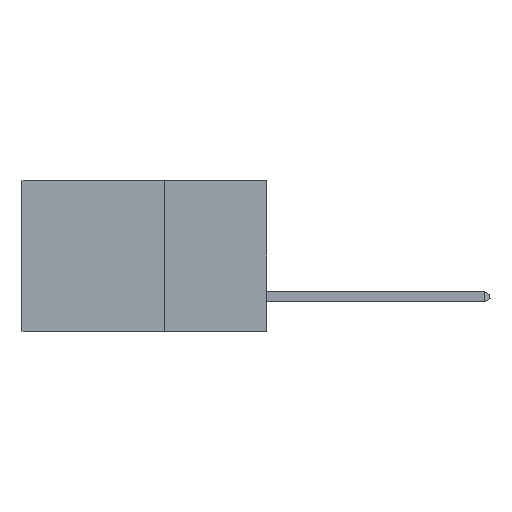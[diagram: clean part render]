
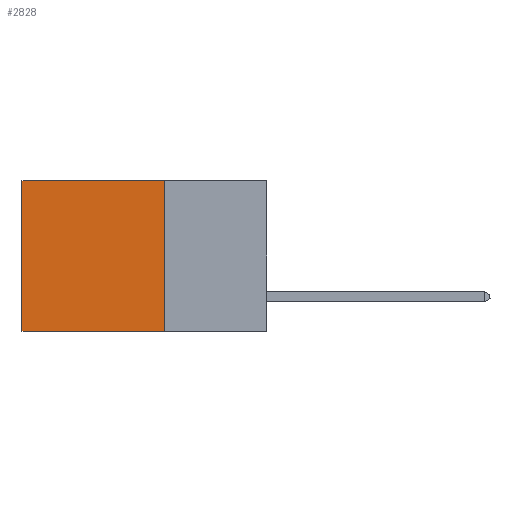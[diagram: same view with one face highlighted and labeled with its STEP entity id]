
A CAD part, left-side view. The second image highlights one B-rep face of the part: STEP entity #2828.
In plain terms, the highlighted planar face has unit normal (-1, 0, 0).
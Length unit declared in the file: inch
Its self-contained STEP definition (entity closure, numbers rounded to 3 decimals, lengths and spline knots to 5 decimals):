
#73 = PLANE ( 'NONE',  #5584 ) ;
#358 = FACE_OUTER_BOUND ( 'NONE', #5738, .T. ) ;
#460 = VERTEX_POINT ( 'NONE', #5154 ) ;
#983 = CARTESIAN_POINT ( 'NONE',  ( 0.2875, 0.25, -0.37 ) ) ;
#1250 = VERTEX_POINT ( 'NONE', #983 ) ;
#1635 = VECTOR ( 'NONE', #7454, 39.37008 ) ;
#1832 = LINE ( 'NONE', #2518, #9228 ) ;
#2518 = CARTESIAN_POINT ( 'NONE',  ( 0.2875, 0.25, 0. ) ) ;
#2676 = VERTEX_POINT ( 'NONE', #5391 ) ;
#2828 = ADVANCED_FACE ( 'NONE', ( #358 ), #73, .F. ) ;
#3034 = EDGE_CURVE ( 'NONE', #1250, #11912, #6338, .T. ) ;
#3839 = DIRECTION ( 'NONE',  ( 0., 1., 0. ) ) ;
#4108 = DIRECTION ( 'NONE',  ( 0., 0., -1. ) ) ;
#4641 = VECTOR ( 'NONE', #10343, 39.37008 ) ;
#5154 = CARTESIAN_POINT ( 'NONE',  ( 0.2875, 0.6, 0. ) ) ;
#5391 = CARTESIAN_POINT ( 'NONE',  ( 0.2875, 0.25, 0. ) ) ;
#5541 = CARTESIAN_POINT ( 'NONE',  ( 0.2875, 0.25, -0.37 ) ) ;
#5584 = AXIS2_PLACEMENT_3D ( 'NONE', #12198, #6181, #4108 ) ;
#5738 = EDGE_LOOP ( 'NONE', ( #9624, #5933, #7737, #12015 ) ) ;
#5933 = ORIENTED_EDGE ( 'NONE', *, *, #3034, .F. ) ;
#6181 = DIRECTION ( 'NONE',  ( 1., 0., 0. ) ) ;
#6338 = LINE ( 'NONE', #5541, #1635 ) ;
#7332 = LINE ( 'NONE', #10415, #4641 ) ;
#7372 = DIRECTION ( 'NONE',  ( 0., 0., -1. ) ) ;
#7454 = DIRECTION ( 'NONE',  ( 0., 1., 0. ) ) ;
#7494 = VECTOR ( 'NONE', #7372, 39.37008 ) ;
#7737 = ORIENTED_EDGE ( 'NONE', *, *, #9472, .F. ) ;
#9228 = VECTOR ( 'NONE', #3839, 39.37008 ) ;
#9324 = EDGE_CURVE ( 'NONE', #2676, #460, #1832, .T. ) ;
#9472 = EDGE_CURVE ( 'NONE', #2676, #1250, #11568, .T. ) ;
#9624 = ORIENTED_EDGE ( 'NONE', *, *, #9854, .T. ) ;
#9854 = EDGE_CURVE ( 'NONE', #460, #11912, #7332, .T. ) ;
#10343 = DIRECTION ( 'NONE',  ( 0., 0., -1. ) ) ;
#10415 = CARTESIAN_POINT ( 'NONE',  ( 0.2875, 0.6, 0. ) ) ;
#11154 = CARTESIAN_POINT ( 'NONE',  ( 0.2875, 0.25, 0. ) ) ;
#11568 = LINE ( 'NONE', #11154, #7494 ) ;
#11912 = VERTEX_POINT ( 'NONE', #12486 ) ;
#12015 = ORIENTED_EDGE ( 'NONE', *, *, #9324, .T. ) ;
#12198 = CARTESIAN_POINT ( 'NONE',  ( 0.2875, 0.25, 0. ) ) ;
#12486 = CARTESIAN_POINT ( 'NONE',  ( 0.2875, 0.6, -0.37 ) ) ;
